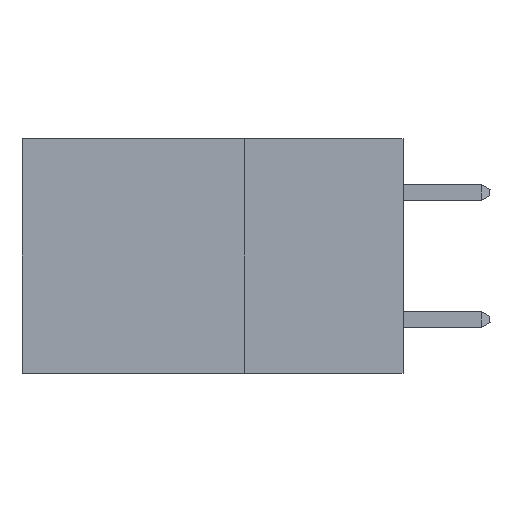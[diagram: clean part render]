
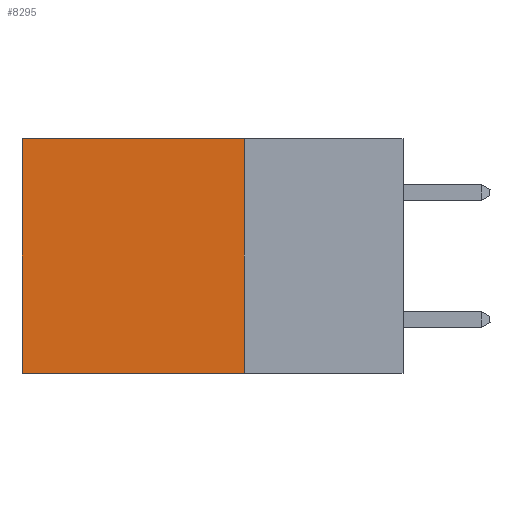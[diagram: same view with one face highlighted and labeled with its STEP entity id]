
A CAD part, left-side view. The second image highlights one B-rep face of the part: STEP entity #8295.
In plain terms, the highlighted planar face has unit normal (-1, 0, 0).
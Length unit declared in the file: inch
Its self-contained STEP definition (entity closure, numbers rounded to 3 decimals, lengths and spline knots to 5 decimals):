
#507 = VERTEX_POINT ( 'NONE', #25870 ) ;
#2369 = CARTESIAN_POINT ( 'NONE',  ( 0.2875, 0.6, 0. ) ) ;
#2945 = CARTESIAN_POINT ( 'NONE',  ( 0.2875, 0.25, 0. ) ) ;
#3881 = AXIS2_PLACEMENT_3D ( 'NONE', #25066, #33857, #16369 ) ;
#4047 = EDGE_CURVE ( 'NONE', #5678, #507, #9256, .T. ) ;
#4777 = EDGE_LOOP ( 'NONE', ( #26536, #11341, #22019, #29504 ) ) ;
#5678 = VERTEX_POINT ( 'NONE', #13975 ) ;
#6102 = DIRECTION ( 'NONE',  ( 0., 1., 0. ) ) ;
#6811 = VECTOR ( 'NONE', #17733, 39.37008 ) ;
#8295 = ADVANCED_FACE ( 'NONE', ( #13753 ), #30943, .F. ) ;
#8476 = DIRECTION ( 'NONE',  ( 0., 0., -1. ) ) ;
#9070 = CARTESIAN_POINT ( 'NONE',  ( 0.2875, 0.25, -0.37 ) ) ;
#9256 = LINE ( 'NONE', #2369, #23984 ) ;
#9412 = EDGE_CURVE ( 'NONE', #34669, #5678, #29689, .T. ) ;
#11341 = ORIENTED_EDGE ( 'NONE', *, *, #18526, .F. ) ;
#13162 = CARTESIAN_POINT ( 'NONE',  ( 0.2875, 0.25, 0. ) ) ;
#13201 = EDGE_CURVE ( 'NONE', #34669, #33141, #37089, .T. ) ;
#13753 = FACE_OUTER_BOUND ( 'NONE', #4777, .T. ) ;
#13975 = CARTESIAN_POINT ( 'NONE',  ( 0.2875, 0.6, 0. ) ) ;
#16369 = DIRECTION ( 'NONE',  ( 0., 0., -1. ) ) ;
#17733 = DIRECTION ( 'NONE',  ( 0., 0., -1. ) ) ;
#18526 = EDGE_CURVE ( 'NONE', #33141, #507, #21633, .T. ) ;
#20822 = CARTESIAN_POINT ( 'NONE',  ( 0.2875, 0.25, -0.37 ) ) ;
#21010 = VECTOR ( 'NONE', #36444, 39.37008 ) ;
#21633 = LINE ( 'NONE', #20822, #26635 ) ;
#22019 = ORIENTED_EDGE ( 'NONE', *, *, #13201, .F. ) ;
#23984 = VECTOR ( 'NONE', #8476, 39.37008 ) ;
#25066 = CARTESIAN_POINT ( 'NONE',  ( 0.2875, 0.25, 0. ) ) ;
#25870 = CARTESIAN_POINT ( 'NONE',  ( 0.2875, 0.6, -0.37 ) ) ;
#26536 = ORIENTED_EDGE ( 'NONE', *, *, #4047, .T. ) ;
#26635 = VECTOR ( 'NONE', #6102, 39.37008 ) ;
#29504 = ORIENTED_EDGE ( 'NONE', *, *, #9412, .T. ) ;
#29689 = LINE ( 'NONE', #13162, #21010 ) ;
#30943 = PLANE ( 'NONE',  #3881 ) ;
#33141 = VERTEX_POINT ( 'NONE', #9070 ) ;
#33225 = CARTESIAN_POINT ( 'NONE',  ( 0.2875, 0.25, 0. ) ) ;
#33857 = DIRECTION ( 'NONE',  ( 1., 0., 0. ) ) ;
#34669 = VERTEX_POINT ( 'NONE', #33225 ) ;
#36444 = DIRECTION ( 'NONE',  ( 0., 1., 0. ) ) ;
#37089 = LINE ( 'NONE', #2945, #6811 ) ;
